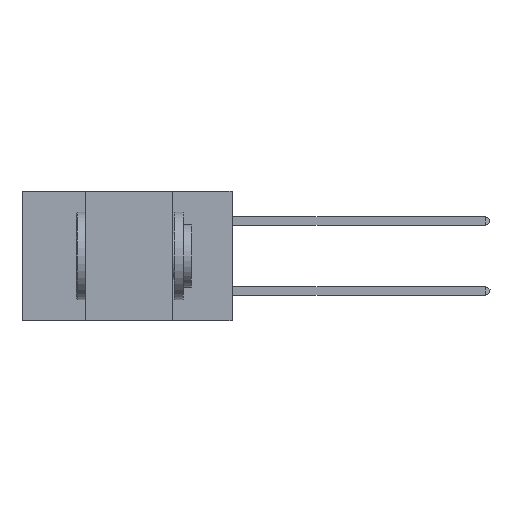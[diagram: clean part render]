
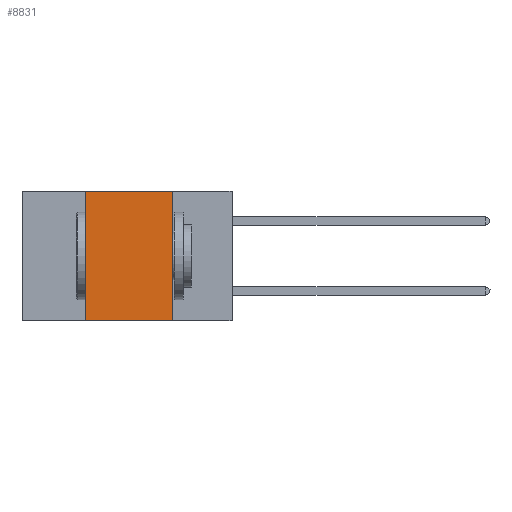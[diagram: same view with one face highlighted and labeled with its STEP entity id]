
A CAD part, left-side view. The second image highlights one B-rep face of the part: STEP entity #8831.
In plain terms, the highlighted planar face has unit normal (-1, 0, 0).
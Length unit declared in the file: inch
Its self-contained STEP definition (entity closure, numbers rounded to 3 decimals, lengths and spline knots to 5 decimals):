
#370 = CARTESIAN_POINT ( 'NONE',  ( 0., 0.42, -0.37 ) ) ;
#514 = VECTOR ( 'NONE', #1388, 39.37008 ) ;
#555 = ORIENTED_EDGE ( 'NONE', *, *, #5437, .F. ) ;
#971 = VERTEX_POINT ( 'NONE', #4599 ) ;
#1169 = VERTEX_POINT ( 'NONE', #5700 ) ;
#1233 = EDGE_CURVE ( 'NONE', #2496, #5280, #7309, .T. ) ;
#1388 = DIRECTION ( 'NONE',  ( 0., -1., 0. ) ) ;
#1461 = VECTOR ( 'NONE', #2846, 39.37008 ) ;
#1604 = DIRECTION ( 'NONE',  ( 1., 0., 0. ) ) ;
#1661 = CARTESIAN_POINT ( 'NONE',  ( 0., 0.42, 0. ) ) ;
#2496 = VERTEX_POINT ( 'NONE', #370 ) ;
#2846 = DIRECTION ( 'NONE',  ( 0., 0., -1. ) ) ;
#2893 = CARTESIAN_POINT ( 'NONE',  ( 0., 0.6, 0. ) ) ;
#3201 = PLANE ( 'NONE',  #8944 ) ;
#3697 = EDGE_CURVE ( 'NONE', #5280, #971, #4757, .T. ) ;
#3855 = ORIENTED_EDGE ( 'NONE', *, *, #1233, .F. ) ;
#4081 = EDGE_LOOP ( 'NONE', ( #555, #6609, #3855, #4526 ) ) ;
#4216 = EDGE_CURVE ( 'NONE', #2496, #1169, #6727, .T. ) ;
#4382 = DIRECTION ( 'NONE',  ( 0., -1., 0. ) ) ;
#4468 = CARTESIAN_POINT ( 'NONE',  ( 0., 0.17, 0. ) ) ;
#4526 = ORIENTED_EDGE ( 'NONE', *, *, #4216, .T. ) ;
#4599 = CARTESIAN_POINT ( 'NONE',  ( 0., 0.17, 0. ) ) ;
#4757 = LINE ( 'NONE', #2893, #514 ) ;
#5280 = VERTEX_POINT ( 'NONE', #5552 ) ;
#5437 = EDGE_CURVE ( 'NONE', #971, #1169, #6961, .T. ) ;
#5552 = CARTESIAN_POINT ( 'NONE',  ( 0., 0.42, 0. ) ) ;
#5700 = CARTESIAN_POINT ( 'NONE',  ( 0., 0.17, -0.37 ) ) ;
#6324 = DIRECTION ( 'NONE',  ( 0., 0., -1. ) ) ;
#6459 = DIRECTION ( 'NONE',  ( 0., 0., 1. ) ) ;
#6597 = VECTOR ( 'NONE', #4382, 39.37008 ) ;
#6609 = ORIENTED_EDGE ( 'NONE', *, *, #3697, .F. ) ;
#6727 = LINE ( 'NONE', #9178, #6597 ) ;
#6927 = VECTOR ( 'NONE', #6459, 39.37008 ) ;
#6961 = LINE ( 'NONE', #4468, #1461 ) ;
#7309 = LINE ( 'NONE', #1661, #6927 ) ;
#8239 = FACE_OUTER_BOUND ( 'NONE', #4081, .T. ) ;
#8795 = CARTESIAN_POINT ( 'NONE',  ( 0., 0.6, 0. ) ) ;
#8831 = ADVANCED_FACE ( 'NONE', ( #8239 ), #3201, .F. ) ;
#8944 = AXIS2_PLACEMENT_3D ( 'NONE', #8795, #1604, #6324 ) ;
#9178 = CARTESIAN_POINT ( 'NONE',  ( 0., 0.6, -0.37 ) ) ;
